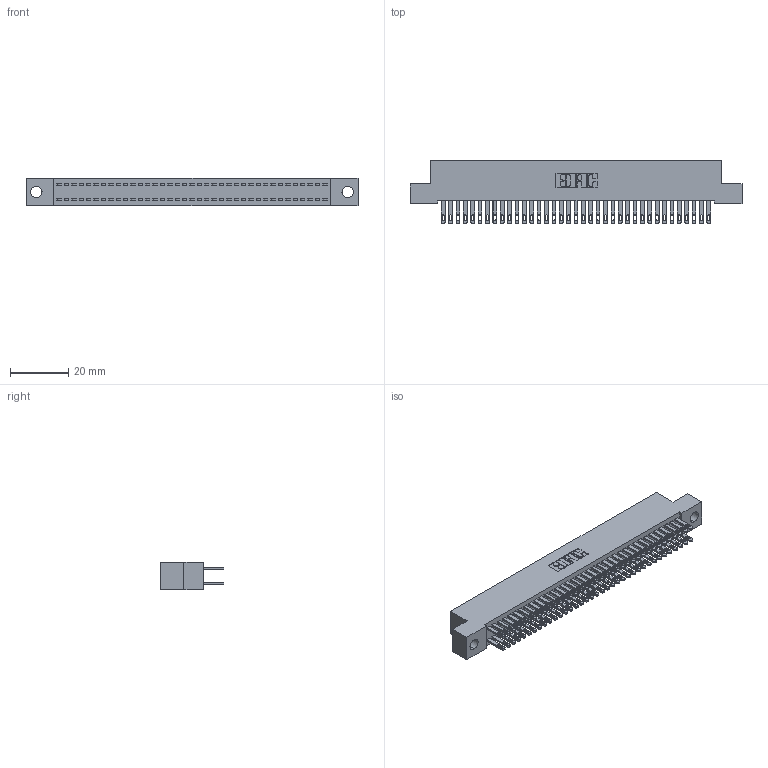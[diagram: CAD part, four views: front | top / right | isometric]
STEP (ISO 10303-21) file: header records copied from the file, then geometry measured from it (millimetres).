
FILE_DESCRIPTION (( 'STEP AP203' ), '1' );
FILE_NAME ('342-074-500-204.STEP', '2019-10-03T16:59:53', ( '' ), ( '' ), 'SwSTEP 2.0', 'SolidWorks 2016', '' );
FILE_SCHEMA (( 'CONFIG_CONTROL_DESIGN' ));
Length unit declared in the file: inch
Products named in the file (3): 342 Part_.156 TH; 345-292-001_345-293-100; 342-074-500-204
Assembly tree (75 placements, depth 2):
  342-074-500-204
    342 Part_.156 TH
    345-292-001_345-293-100  x74
Bounding box: 114.3 x 21.85 x 9.4 mm (x, y, z)
Volume: 10385.3 mm3; surface area: 17314.1 mm2
Topology: 75 solids, 75 shells, 3662 faces, 11177 edges, 7450 vertices
Faces by surface type: plane 2286, cylinder 1376
Entity records: 24251 total; most frequent: CARTESIAN_POINT 4022, ORIENTED_EDGE 3958, DIRECTION 3447, EDGE_CURVE 1979, VECTOR 1847, LINE 1847, VERTEX_POINT 1318, AXIS2_PLACEMENT_3D 800
